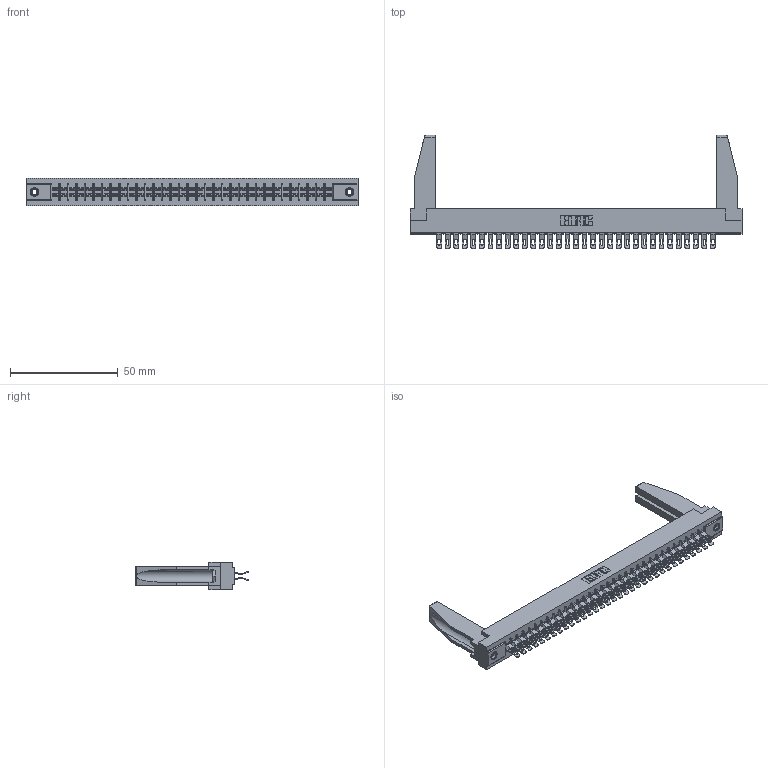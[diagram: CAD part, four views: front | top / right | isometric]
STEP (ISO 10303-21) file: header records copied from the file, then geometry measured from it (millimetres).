
FILE_DESCRIPTION (( 'STEP AP203' ), '1' );
FILE_NAME ('305-066-555-578.STEP', '2019-09-10T03:50:34', ( '' ), ( '' ), 'SwSTEP 2.0', 'SolidWorks 2016', '' );
FILE_SCHEMA (( 'CONFIG_CONTROL_DESIGN' ));
Length unit declared in the file: inch
Products named in the file (5): 305 Part_.156 Dia; 305-290-001_555; 305-066-555-578; 345-250-001_345-250-001-102; 307-220-078
Assembly tree (71 placements, depth 2):
  305-066-555-578
    305 Part_.156 Dia
    305-290-001_555  x66
    345-250-001_345-250-001-102  x2
    307-220-078  x2
Bounding box: 153.77 x 52.45 x 12.7 mm (x, y, z)
Volume: 19719.4 mm3; surface area: 25602.6 mm2
Topology: 71 solids, 71 shells, 4602 faces, 13681 edges, 8934 vertices
Faces by surface type: plane 2264, cylinder 2190, sphere 132, cone 12, torus 4
Entity records: 39889 total; most frequent: CARTESIAN_POINT 6625, ORIENTED_EDGE 6524, DIRECTION 6368, EDGE_CURVE 3262, VECTOR 2606, LINE 2606, VERTEX_POINT 2080, AXIS2_PLACEMENT_3D 1881
